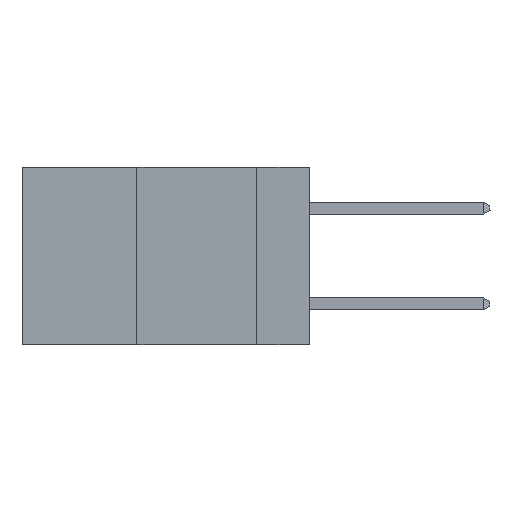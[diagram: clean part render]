
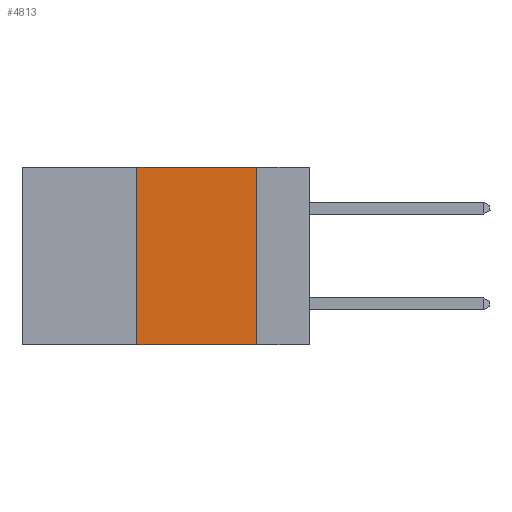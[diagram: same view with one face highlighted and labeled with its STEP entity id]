
A CAD part, left-side view. The second image highlights one B-rep face of the part: STEP entity #4813.
In plain terms, the highlighted planar face has unit normal (-1, 0, 0).
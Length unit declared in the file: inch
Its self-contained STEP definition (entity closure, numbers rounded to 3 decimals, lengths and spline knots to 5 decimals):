
#235 = DIRECTION ( 'NONE',  ( 0., -1., 0. ) ) ;
#454 = CARTESIAN_POINT ( 'NONE',  ( 0., 0.6, -0.37 ) ) ;
#2724 = ORIENTED_EDGE ( 'NONE', *, *, #23261, .F. ) ;
#2799 = FACE_OUTER_BOUND ( 'NONE', #8128, .T. ) ;
#3370 = AXIS2_PLACEMENT_3D ( 'NONE', #24128, #29903, #15188 ) ;
#4488 = EDGE_CURVE ( 'NONE', #37368, #10478, #12624, .T. ) ;
#4813 = ADVANCED_FACE ( 'NONE', ( #2799 ), #11998, .F. ) ;
#7706 = VECTOR ( 'NONE', #37551, 39.37008 ) ;
#8128 = EDGE_LOOP ( 'NONE', ( #21241, #25153, #2724, #28413 ) ) ;
#9083 = VECTOR ( 'NONE', #9600, 39.37008 ) ;
#9600 = DIRECTION ( 'NONE',  ( 0., -1., 0. ) ) ;
#9984 = CARTESIAN_POINT ( 'NONE',  ( 0., 0.6, 0. ) ) ;
#10478 = VERTEX_POINT ( 'NONE', #31296 ) ;
#11510 = CARTESIAN_POINT ( 'NONE',  ( 0., 0.36, 0. ) ) ;
#11998 = PLANE ( 'NONE',  #3370 ) ;
#12624 = LINE ( 'NONE', #454, #9083 ) ;
#15188 = DIRECTION ( 'NONE',  ( 0., 0., -1. ) ) ;
#21241 = ORIENTED_EDGE ( 'NONE', *, *, #39355, .F. ) ;
#21742 = CARTESIAN_POINT ( 'NONE',  ( 0., 0.11, 0. ) ) ;
#21840 = CARTESIAN_POINT ( 'NONE',  ( 0., 0.36, -0.37 ) ) ;
#21946 = LINE ( 'NONE', #9984, #37443 ) ;
#22422 = VERTEX_POINT ( 'NONE', #21742 ) ;
#23261 = EDGE_CURVE ( 'NONE', #37368, #26412, #23276, .T. ) ;
#23276 = LINE ( 'NONE', #11510, #35528 ) ;
#24128 = CARTESIAN_POINT ( 'NONE',  ( 0., 0.6, 0. ) ) ;
#24974 = CARTESIAN_POINT ( 'NONE',  ( 0., 0.11, 0. ) ) ;
#25153 = ORIENTED_EDGE ( 'NONE', *, *, #31761, .F. ) ;
#25369 = LINE ( 'NONE', #24974, #7706 ) ;
#26412 = VERTEX_POINT ( 'NONE', #34074 ) ;
#28413 = ORIENTED_EDGE ( 'NONE', *, *, #4488, .T. ) ;
#29644 = DIRECTION ( 'NONE',  ( 0., 0., 1. ) ) ;
#29903 = DIRECTION ( 'NONE',  ( 1., 0., 0. ) ) ;
#31296 = CARTESIAN_POINT ( 'NONE',  ( 0., 0.11, -0.37 ) ) ;
#31761 = EDGE_CURVE ( 'NONE', #26412, #22422, #21946, .T. ) ;
#34074 = CARTESIAN_POINT ( 'NONE',  ( 0., 0.36, 0. ) ) ;
#35528 = VECTOR ( 'NONE', #29644, 39.37008 ) ;
#37368 = VERTEX_POINT ( 'NONE', #21840 ) ;
#37443 = VECTOR ( 'NONE', #235, 39.37008 ) ;
#37551 = DIRECTION ( 'NONE',  ( 0., 0., -1. ) ) ;
#39355 = EDGE_CURVE ( 'NONE', #22422, #10478, #25369, .T. ) ;
